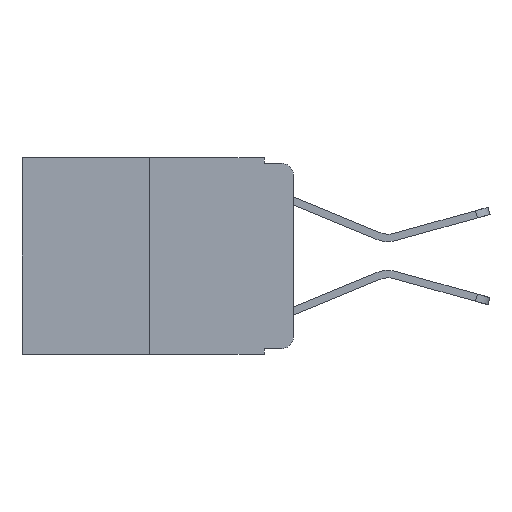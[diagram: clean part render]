
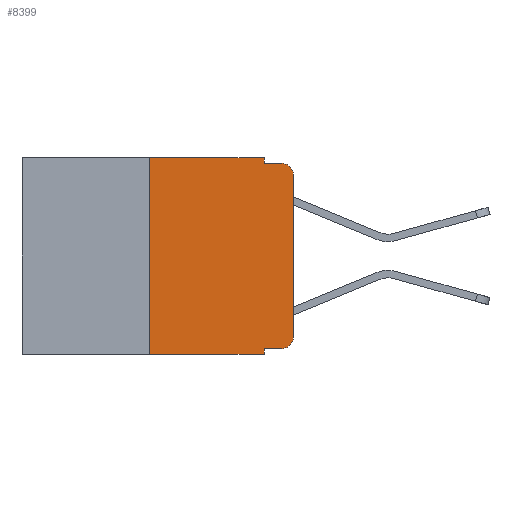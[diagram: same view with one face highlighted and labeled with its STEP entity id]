
A CAD part, left-side view. The second image highlights one B-rep face of the part: STEP entity #8399.
In plain terms, the highlighted planar face has unit normal (-1, 0, 0).
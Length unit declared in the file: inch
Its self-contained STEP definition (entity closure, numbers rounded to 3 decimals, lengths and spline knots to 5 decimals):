
#3 = ORIENTED_EDGE ( 'NONE', *, *, #14839, .T. ) ;
#49 = ORIENTED_EDGE ( 'NONE', *, *, #1623, .F. ) ;
#218 = DIRECTION ( 'NONE',  ( -1., 0., 0. ) ) ;
#480 = AXIS2_PLACEMENT_3D ( 'NONE', #13795, #3427, #15433 ) ;
#619 = AXIS2_PLACEMENT_3D ( 'NONE', #17481, #16003, #5818 ) ;
#952 = CARTESIAN_POINT ( 'NONE',  ( 0., 0., -0.313 ) ) ;
#1000 = VERTEX_POINT ( 'NONE', #17812 ) ;
#1071 = ORIENTED_EDGE ( 'NONE', *, *, #16995, .F. ) ;
#1272 = ORIENTED_EDGE ( 'NONE', *, *, #21866, .T. ) ;
#1406 = VERTEX_POINT ( 'NONE', #14027 ) ;
#1623 = EDGE_CURVE ( 'NONE', #1406, #13419, #5721, .T. ) ;
#1676 = DIRECTION ( 'NONE',  ( 0., 0., -1. ) ) ;
#1680 = CARTESIAN_POINT ( 'NONE',  ( 0., 0.473, 0. ) ) ;
#2668 = CARTESIAN_POINT ( 'NONE',  ( 0., 0.051, 0. ) ) ;
#2677 = ORIENTED_EDGE ( 'NONE', *, *, #11136, .T. ) ;
#3010 = VERTEX_POINT ( 'NONE', #15091 ) ;
#3427 = DIRECTION ( 'NONE',  ( -1., 0., 0. ) ) ;
#3594 = EDGE_CURVE ( 'NONE', #20455, #3010, #8418, .T. ) ;
#4036 = PLANE ( 'NONE',  #619 ) ;
#4249 = CIRCLE ( 'NONE', #480, 0.02 ) ;
#5170 = FACE_OUTER_BOUND ( 'NONE', #12210, .T. ) ;
#5285 = DIRECTION ( 'NONE',  ( 0., -1., 0. ) ) ;
#5721 = LINE ( 'NONE', #13928, #10956 ) ;
#5812 = CARTESIAN_POINT ( 'NONE',  ( 0., 0.25, -0.343 ) ) ;
#5818 = DIRECTION ( 'NONE',  ( 0., 0., -1. ) ) ;
#6026 = LINE ( 'NONE', #21768, #13575 ) ;
#6374 = CARTESIAN_POINT ( 'NONE',  ( 0., 0.051, -0.01 ) ) ;
#6704 = AXIS2_PLACEMENT_3D ( 'NONE', #10868, #218, #12542 ) ;
#6745 = CIRCLE ( 'NONE', #6704, 0.02 ) ;
#7879 = EDGE_CURVE ( 'NONE', #1000, #16297, #12017, .T. ) ;
#8002 = DIRECTION ( 'NONE',  ( 0., 0., -1. ) ) ;
#8399 = ADVANCED_FACE ( 'NONE', ( #5170 ), #4036, .F. ) ;
#8418 = LINE ( 'NONE', #18185, #12464 ) ;
#9000 = LINE ( 'NONE', #17971, #13518 ) ;
#9062 = DIRECTION ( 'NONE',  ( 0., -1., 0. ) ) ;
#9120 = EDGE_CURVE ( 'NONE', #20455, #16297, #9000, .T. ) ;
#9410 = ORIENTED_EDGE ( 'NONE', *, *, #16894, .F. ) ;
#9790 = ORIENTED_EDGE ( 'NONE', *, *, #18726, .T. ) ;
#9962 = DIRECTION ( 'NONE',  ( 0., -1., 0. ) ) ;
#10098 = CARTESIAN_POINT ( 'NONE',  ( 0., 0.02, -0.01 ) ) ;
#10220 = DIRECTION ( 'NONE',  ( 0., 0., 1. ) ) ;
#10868 = CARTESIAN_POINT ( 'NONE',  ( 0., 0.02, -0.03 ) ) ;
#10956 = VECTOR ( 'NONE', #1676, 39.37008 ) ;
#11100 = VERTEX_POINT ( 'NONE', #952 ) ;
#11136 = EDGE_CURVE ( 'NONE', #1000, #16958, #17767, .T. ) ;
#11217 = VERTEX_POINT ( 'NONE', #10098 ) ;
#11227 = ORIENTED_EDGE ( 'NONE', *, *, #7879, .F. ) ;
#11594 = CARTESIAN_POINT ( 'NONE',  ( 0., 0.051, -0.333 ) ) ;
#12017 = LINE ( 'NONE', #2668, #14845 ) ;
#12210 = EDGE_LOOP ( 'NONE', ( #1272, #3, #1071, #49, #9410, #14827, #15700, #11227, #2677, #9790 ) ) ;
#12464 = VECTOR ( 'NONE', #18031, 39.37008 ) ;
#12542 = DIRECTION ( 'NONE',  ( 0., 0., -1. ) ) ;
#13120 = VERTEX_POINT ( 'NONE', #15604 ) ;
#13387 = LINE ( 'NONE', #1680, #21606 ) ;
#13419 = VERTEX_POINT ( 'NONE', #6374 ) ;
#13459 = VECTOR ( 'NONE', #9962, 39.37008 ) ;
#13518 = VECTOR ( 'NONE', #19680, 39.37008 ) ;
#13575 = VECTOR ( 'NONE', #10220, 39.37008 ) ;
#13795 = CARTESIAN_POINT ( 'NONE',  ( 0., 0.02, -0.313 ) ) ;
#13928 = CARTESIAN_POINT ( 'NONE',  ( 0., 0.051, 0. ) ) ;
#14027 = CARTESIAN_POINT ( 'NONE',  ( 0., 0.051, 0. ) ) ;
#14827 = ORIENTED_EDGE ( 'NONE', *, *, #3594, .F. ) ;
#14839 = EDGE_CURVE ( 'NONE', #13120, #11217, #6745, .T. ) ;
#14845 = VECTOR ( 'NONE', #8002, 39.37008 ) ;
#15091 = CARTESIAN_POINT ( 'NONE',  ( 0., 0.25, 0. ) ) ;
#15168 = VECTOR ( 'NONE', #9062, 39.37008 ) ;
#15433 = DIRECTION ( 'NONE',  ( 0., 0., -1. ) ) ;
#15604 = CARTESIAN_POINT ( 'NONE',  ( 0., 0., -0.03 ) ) ;
#15673 = LINE ( 'NONE', #17401, #15168 ) ;
#15700 = ORIENTED_EDGE ( 'NONE', *, *, #9120, .T. ) ;
#15712 = CARTESIAN_POINT ( 'NONE',  ( 0., 0.02, -0.333 ) ) ;
#16003 = DIRECTION ( 'NONE',  ( 1., 0., 0. ) ) ;
#16297 = VERTEX_POINT ( 'NONE', #18593 ) ;
#16894 = EDGE_CURVE ( 'NONE', #3010, #1406, #13387, .T. ) ;
#16958 = VERTEX_POINT ( 'NONE', #15712 ) ;
#16995 = EDGE_CURVE ( 'NONE', #13419, #11217, #15673, .T. ) ;
#17401 = CARTESIAN_POINT ( 'NONE',  ( 0., 0.051, -0.01 ) ) ;
#17481 = CARTESIAN_POINT ( 'NONE',  ( 0., 0.473, 0. ) ) ;
#17767 = LINE ( 'NONE', #11594, #13459 ) ;
#17812 = CARTESIAN_POINT ( 'NONE',  ( 0., 0.051, -0.333 ) ) ;
#17971 = CARTESIAN_POINT ( 'NONE',  ( 0., 0.473, -0.343 ) ) ;
#18031 = DIRECTION ( 'NONE',  ( 0., 0., 1. ) ) ;
#18185 = CARTESIAN_POINT ( 'NONE',  ( 0., 0.25, 0. ) ) ;
#18593 = CARTESIAN_POINT ( 'NONE',  ( 0., 0.051, -0.343 ) ) ;
#18726 = EDGE_CURVE ( 'NONE', #16958, #11100, #4249, .T. ) ;
#19680 = DIRECTION ( 'NONE',  ( 0., -1., 0. ) ) ;
#20455 = VERTEX_POINT ( 'NONE', #5812 ) ;
#21606 = VECTOR ( 'NONE', #5285, 39.37008 ) ;
#21768 = CARTESIAN_POINT ( 'NONE',  ( 0., 0., 0. ) ) ;
#21866 = EDGE_CURVE ( 'NONE', #11100, #13120, #6026, .T. ) ;
